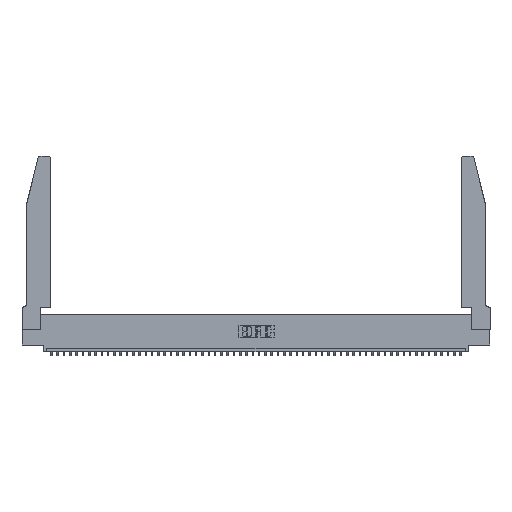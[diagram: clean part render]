
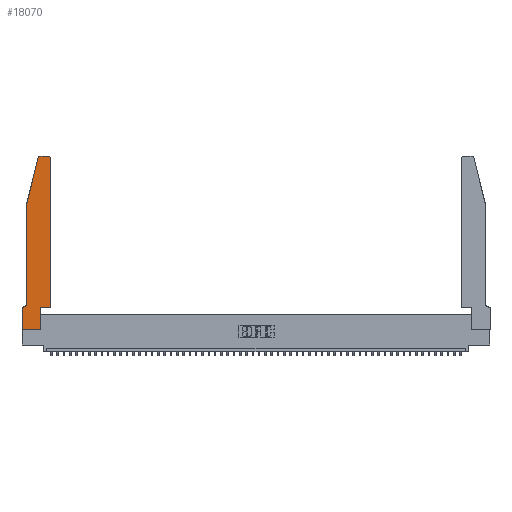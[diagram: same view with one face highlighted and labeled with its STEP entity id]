
A CAD part, top view. The second image highlights one B-rep face of the part: STEP entity #18070.
In plain terms, the highlighted planar face has unit normal (0, 0, 1).
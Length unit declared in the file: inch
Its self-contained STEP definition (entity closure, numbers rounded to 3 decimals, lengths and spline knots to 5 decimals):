
#735 = VECTOR ( 'NONE', #19140, 39.37008 ) ;
#1566 = DIRECTION ( 'NONE',  ( -1., 0., 0. ) ) ;
#1717 = CARTESIAN_POINT ( 'NONE',  ( 0., 0., 0.37 ) ) ;
#2228 = CARTESIAN_POINT ( 'NONE',  ( 0., 0., 0.37 ) ) ;
#2239 = VERTEX_POINT ( 'NONE', #14697 ) ;
#3885 = AXIS2_PLACEMENT_3D ( 'NONE', #21064, #48844, #5254 ) ;
#4161 = VERTEX_POINT ( 'NONE', #43645 ) ;
#4312 = VERTEX_POINT ( 'NONE', #13378 ) ;
#5254 = DIRECTION ( 'NONE',  ( 1., 0., 0. ) ) ;
#5332 = ORIENTED_EDGE ( 'NONE', *, *, #36706, .T. ) ;
#5551 = CARTESIAN_POINT ( 'NONE',  ( 0.2865, 0., 0.37 ) ) ;
#7254 = LINE ( 'NONE', #34597, #35810 ) ;
#7397 = VERTEX_POINT ( 'NONE', #19200 ) ;
#7729 = CARTESIAN_POINT ( 'NONE',  ( 0.4205, 2.72, 0.37 ) ) ;
#9504 = LINE ( 'NONE', #2228, #12598 ) ;
#9963 = ORIENTED_EDGE ( 'NONE', *, *, #42682, .T. ) ;
#10065 = DIRECTION ( 'NONE',  ( 0., 0., -1. ) ) ;
#10371 = EDGE_CURVE ( 'NONE', #2239, #49654, #17349, .T. ) ;
#10501 = VERTEX_POINT ( 'NONE', #18631 ) ;
#10613 = DIRECTION ( 'NONE',  ( 0., 1., 0. ) ) ;
#11015 = LINE ( 'NONE', #45184, #15969 ) ;
#11517 = ORIENTED_EDGE ( 'NONE', *, *, #41927, .T. ) ;
#12333 = DIRECTION ( 'NONE',  ( 1., 0., 0. ) ) ;
#12598 = VECTOR ( 'NONE', #45378, 39.37008 ) ;
#12943 = CARTESIAN_POINT ( 'NONE',  ( 0.0755, 0.35, 0.37 ) ) ;
#13378 = CARTESIAN_POINT ( 'NONE',  ( 0.25487, 2.72718, 0.37 ) ) ;
#13790 = LINE ( 'NONE', #38937, #735 ) ;
#14397 = ORIENTED_EDGE ( 'NONE', *, *, #34395, .T. ) ;
#14403 = VERTEX_POINT ( 'NONE', #30252 ) ;
#14697 = CARTESIAN_POINT ( 'NONE',  ( 0.4205, 2.75, 0.37 ) ) ;
#15222 = CARTESIAN_POINT ( 'NONE',  ( 0., 0., 0.37 ) ) ;
#15969 = VECTOR ( 'NONE', #49068, 39.37008 ) ;
#16990 = CARTESIAN_POINT ( 'NONE',  ( 0.0755, 2., 0.37 ) ) ;
#17046 = CARTESIAN_POINT ( 'NONE',  ( 0.4505, 2.72, 0.37 ) ) ;
#17153 = EDGE_CURVE ( 'NONE', #51355, #4161, #49657, .T. ) ;
#17339 = CARTESIAN_POINT ( 'NONE',  ( 0.284, 2.72, 0.37 ) ) ;
#17349 = LINE ( 'NONE', #26366, #32816 ) ;
#17466 = ORIENTED_EDGE ( 'NONE', *, *, #48129, .T. ) ;
#18070 = ADVANCED_FACE ( 'NONE', ( #18116 ), #44823, .T. ) ;
#18116 = FACE_OUTER_BOUND ( 'NONE', #38526, .T. ) ;
#18631 = CARTESIAN_POINT ( 'NONE',  ( 0.0755, 0.42, 0.37 ) ) ;
#18913 = VECTOR ( 'NONE', #27239, 39.37008 ) ;
#19140 = DIRECTION ( 'NONE',  ( -0.239, -0.971, 0. ) ) ;
#19200 = CARTESIAN_POINT ( 'NONE',  ( 0.0055, 0.35, 0.37 ) ) ;
#20754 = LINE ( 'NONE', #1717, #18913 ) ;
#21064 = CARTESIAN_POINT ( 'NONE',  ( 0., 0.35, 0.37 ) ) ;
#22657 = AXIS2_PLACEMENT_3D ( 'NONE', #7729, #39306, #43624 ) ;
#22745 = CARTESIAN_POINT ( 'NONE',  ( 0.2865, 0.35, 0.37 ) ) ;
#22811 = CARTESIAN_POINT ( 'NONE',  ( 0.4505, 0.35, 0.37 ) ) ;
#24207 = EDGE_CURVE ( 'NONE', #36115, #48457, #38922, .T. ) ;
#24587 = VECTOR ( 'NONE', #26475, 39.37008 ) ;
#25696 = CARTESIAN_POINT ( 'NONE',  ( 0.4505, 0.35, 0.37 ) ) ;
#26366 = CARTESIAN_POINT ( 'NONE',  ( 0.2605, 2.75, 0.37 ) ) ;
#26475 = DIRECTION ( 'NONE',  ( 0., 1., 0. ) ) ;
#27056 = AXIS2_PLACEMENT_3D ( 'NONE', #33839, #10065, #49290 ) ;
#27239 = DIRECTION ( 'NONE',  ( 1., 0., 0. ) ) ;
#27314 = CIRCLE ( 'NONE', #38314, 0.03 ) ;
#28169 = EDGE_CURVE ( 'NONE', #35314, #51355, #20754, .T. ) ;
#28489 = VECTOR ( 'NONE', #10613, 39.37008 ) ;
#28914 = ORIENTED_EDGE ( 'NONE', *, *, #43784, .T. ) ;
#29383 = ORIENTED_EDGE ( 'NONE', *, *, #24207, .T. ) ;
#30252 = CARTESIAN_POINT ( 'NONE',  ( 0., 0.35, 0.37 ) ) ;
#32816 = VECTOR ( 'NONE', #1566, 39.37008 ) ;
#33460 = CIRCLE ( 'NONE', #27056, 0.07 ) ;
#33473 = DIRECTION ( 'NONE',  ( 1., 0., 0. ) ) ;
#33839 = CARTESIAN_POINT ( 'NONE',  ( 0.0055, 0.42, 0.37 ) ) ;
#34253 = VERTEX_POINT ( 'NONE', #16990 ) ;
#34395 = EDGE_CURVE ( 'NONE', #4161, #36115, #7254, .T. ) ;
#34597 = CARTESIAN_POINT ( 'NONE',  ( 0.4505, 0.35, 0.37 ) ) ;
#34799 = ORIENTED_EDGE ( 'NONE', *, *, #10371, .T. ) ;
#35314 = VERTEX_POINT ( 'NONE', #15222 ) ;
#35810 = VECTOR ( 'NONE', #12333, 39.37008 ) ;
#36115 = VERTEX_POINT ( 'NONE', #25696 ) ;
#36706 = EDGE_CURVE ( 'NONE', #7397, #14403, #51097, .T. ) ;
#37071 = DIRECTION ( 'NONE',  ( -1., 0., 0. ) ) ;
#38034 = VECTOR ( 'NONE', #37071, 39.37008 ) ;
#38314 = AXIS2_PLACEMENT_3D ( 'NONE', #17339, #48921, #33473 ) ;
#38526 = EDGE_LOOP ( 'NONE', ( #34799, #40828, #9963, #28914, #42398, #5332, #11517, #45948, #47146, #14397, #29383, #17466 ) ) ;
#38922 = LINE ( 'NONE', #22811, #24587 ) ;
#38937 = CARTESIAN_POINT ( 'NONE',  ( 0.0755, 2., 0.37 ) ) ;
#39098 = EDGE_CURVE ( 'NONE', #10501, #7397, #33460, .T. ) ;
#39306 = DIRECTION ( 'NONE',  ( 0., 0., 1. ) ) ;
#40828 = ORIENTED_EDGE ( 'NONE', *, *, #49117, .T. ) ;
#41642 = CIRCLE ( 'NONE', #22657, 0.03 ) ;
#41927 = EDGE_CURVE ( 'NONE', #14403, #35314, #9504, .T. ) ;
#42398 = ORIENTED_EDGE ( 'NONE', *, *, #39098, .T. ) ;
#42682 = EDGE_CURVE ( 'NONE', #4312, #34253, #13790, .T. ) ;
#43624 = DIRECTION ( 'NONE',  ( 1., 0., 0. ) ) ;
#43645 = CARTESIAN_POINT ( 'NONE',  ( 0.2865, 0.35, 0.37 ) ) ;
#43784 = EDGE_CURVE ( 'NONE', #34253, #10501, #11015, .T. ) ;
#44823 = PLANE ( 'NONE',  #3885 ) ;
#45184 = CARTESIAN_POINT ( 'NONE',  ( 0.0755, 2., 0.37 ) ) ;
#45378 = DIRECTION ( 'NONE',  ( 0., -1., 0. ) ) ;
#45948 = ORIENTED_EDGE ( 'NONE', *, *, #28169, .T. ) ;
#47146 = ORIENTED_EDGE ( 'NONE', *, *, #17153, .T. ) ;
#48129 = EDGE_CURVE ( 'NONE', #48457, #2239, #41642, .T. ) ;
#48457 = VERTEX_POINT ( 'NONE', #17046 ) ;
#48519 = CARTESIAN_POINT ( 'NONE',  ( 0.284, 2.75, 0.37 ) ) ;
#48844 = DIRECTION ( 'NONE',  ( 0., 0., 1. ) ) ;
#48921 = DIRECTION ( 'NONE',  ( 0., 0., 1. ) ) ;
#49068 = DIRECTION ( 'NONE',  ( 0., -1., 0. ) ) ;
#49117 = EDGE_CURVE ( 'NONE', #49654, #4312, #27314, .T. ) ;
#49290 = DIRECTION ( 'NONE',  ( -1., 0., 0. ) ) ;
#49654 = VERTEX_POINT ( 'NONE', #48519 ) ;
#49657 = LINE ( 'NONE', #22745, #28489 ) ;
#51097 = LINE ( 'NONE', #12943, #38034 ) ;
#51355 = VERTEX_POINT ( 'NONE', #5551 ) ;
